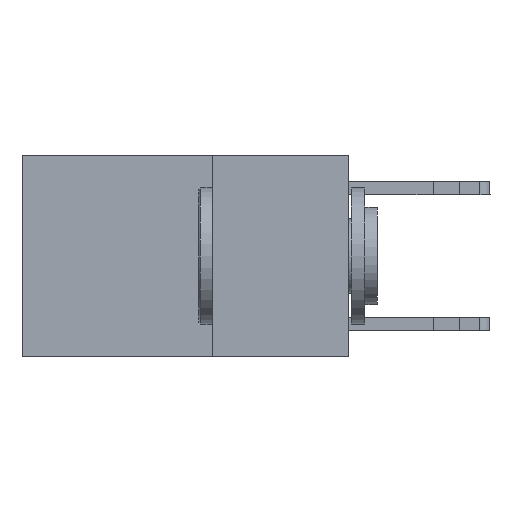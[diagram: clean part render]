
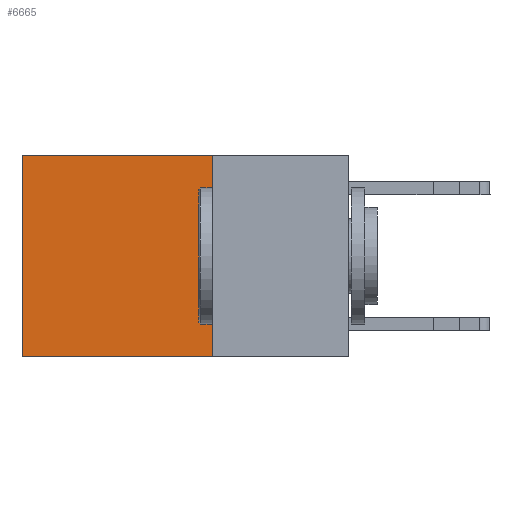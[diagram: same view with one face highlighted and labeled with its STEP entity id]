
A CAD part, left-side view. The second image highlights one B-rep face of the part: STEP entity #6665.
In plain terms, the highlighted planar face has unit normal (-1, 0, 0).
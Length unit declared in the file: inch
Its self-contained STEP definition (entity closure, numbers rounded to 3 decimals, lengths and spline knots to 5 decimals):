
#600 = DIRECTION ( 'NONE',  ( 0., 1., 0. ) ) ;
#912 = CARTESIAN_POINT ( 'NONE',  ( 0.2625, 0.25, -0.37 ) ) ;
#1558 = DIRECTION ( 'NONE',  ( 1., 0., 0. ) ) ;
#1870 = DIRECTION ( 'NONE',  ( 0., 0., -1. ) ) ;
#1945 = VECTOR ( 'NONE', #19636, 39.37008 ) ;
#5070 = VECTOR ( 'NONE', #7979, 39.37008 ) ;
#5749 = EDGE_CURVE ( 'NONE', #6902, #13837, #12917, .T. ) ;
#6494 = CARTESIAN_POINT ( 'NONE',  ( 0.2625, 0.6, 0. ) ) ;
#6532 = AXIS2_PLACEMENT_3D ( 'NONE', #17163, #1558, #1870 ) ;
#6553 = CARTESIAN_POINT ( 'NONE',  ( 0.2625, 0.6, 0. ) ) ;
#6592 = ORIENTED_EDGE ( 'NONE', *, *, #12903, .T. ) ;
#6665 = ADVANCED_FACE ( 'NONE', ( #11851 ), #18750, .F. ) ;
#6780 = ORIENTED_EDGE ( 'NONE', *, *, #5749, .F. ) ;
#6902 = VERTEX_POINT ( 'NONE', #11122 ) ;
#7041 = CARTESIAN_POINT ( 'NONE',  ( 0.2625, 0.6, -0.37 ) ) ;
#7128 = VECTOR ( 'NONE', #17220, 39.37008 ) ;
#7364 = LINE ( 'NONE', #19297, #1945 ) ;
#7979 = DIRECTION ( 'NONE',  ( 0., 1., 0. ) ) ;
#9934 = EDGE_LOOP ( 'NONE', ( #6592, #6780, #17353, #20779 ) ) ;
#10014 = LINE ( 'NONE', #6553, #7128 ) ;
#11036 = CARTESIAN_POINT ( 'NONE',  ( 0.2625, 0.25, 0. ) ) ;
#11122 = CARTESIAN_POINT ( 'NONE',  ( 0.2625, 0.25, -0.37 ) ) ;
#11127 = VERTEX_POINT ( 'NONE', #11036 ) ;
#11851 = FACE_OUTER_BOUND ( 'NONE', #9934, .T. ) ;
#12482 = EDGE_CURVE ( 'NONE', #11127, #21318, #16110, .T. ) ;
#12903 = EDGE_CURVE ( 'NONE', #21318, #13837, #10014, .T. ) ;
#12917 = LINE ( 'NONE', #912, #5070 ) ;
#13837 = VERTEX_POINT ( 'NONE', #7041 ) ;
#16110 = LINE ( 'NONE', #21207, #20825 ) ;
#17163 = CARTESIAN_POINT ( 'NONE',  ( 0.2625, 0.25, 0. ) ) ;
#17220 = DIRECTION ( 'NONE',  ( 0., 0., -1. ) ) ;
#17353 = ORIENTED_EDGE ( 'NONE', *, *, #20143, .F. ) ;
#18750 = PLANE ( 'NONE',  #6532 ) ;
#19297 = CARTESIAN_POINT ( 'NONE',  ( 0.2625, 0.25, 0. ) ) ;
#19636 = DIRECTION ( 'NONE',  ( 0., 0., -1. ) ) ;
#20143 = EDGE_CURVE ( 'NONE', #11127, #6902, #7364, .T. ) ;
#20779 = ORIENTED_EDGE ( 'NONE', *, *, #12482, .T. ) ;
#20825 = VECTOR ( 'NONE', #600, 39.37008 ) ;
#21207 = CARTESIAN_POINT ( 'NONE',  ( 0.2625, 0.25, 0. ) ) ;
#21318 = VERTEX_POINT ( 'NONE', #6494 ) ;
